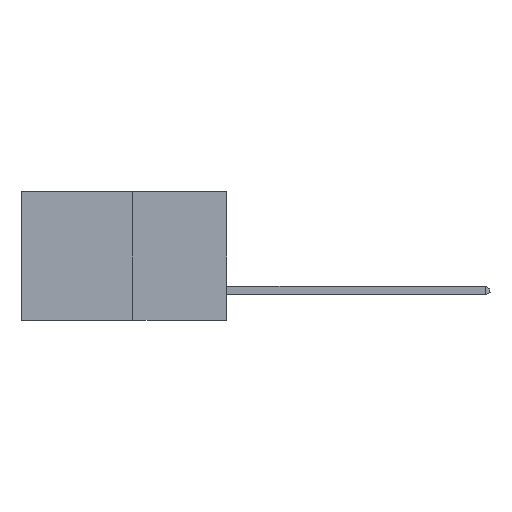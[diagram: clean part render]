
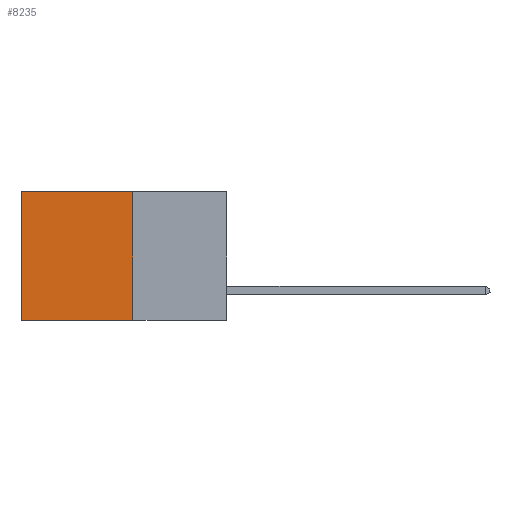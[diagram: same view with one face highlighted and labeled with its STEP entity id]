
A CAD part, left-side view. The second image highlights one B-rep face of the part: STEP entity #8235.
In plain terms, the highlighted planar face has unit normal (-1, 0, 0).
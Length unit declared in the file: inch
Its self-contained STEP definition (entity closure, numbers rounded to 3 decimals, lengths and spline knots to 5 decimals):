
#648 = LINE ( 'NONE', #4608, #25871 ) ;
#2080 = CARTESIAN_POINT ( 'NONE',  ( 0.277, 0.27, 0. ) ) ;
#4312 = VERTEX_POINT ( 'NONE', #30359 ) ;
#4608 = CARTESIAN_POINT ( 'NONE',  ( 0.277, 0.59, -0.37 ) ) ;
#6046 = PLANE ( 'NONE',  #11233 ) ;
#8235 = ADVANCED_FACE ( 'NONE', ( #15177 ), #6046, .F. ) ;
#8354 = EDGE_CURVE ( 'NONE', #21498, #4312, #23986, .T. ) ;
#8487 = DIRECTION ( 'NONE',  ( 1., 0., 0. ) ) ;
#8508 = CARTESIAN_POINT ( 'NONE',  ( 0.277, 0.27, -0.37 ) ) ;
#10447 = ORIENTED_EDGE ( 'NONE', *, *, #8354, .F. ) ;
#10821 = CARTESIAN_POINT ( 'NONE',  ( 0.277, 0.27, -0.37 ) ) ;
#10945 = DIRECTION ( 'NONE',  ( 0., 0., -1. ) ) ;
#11233 = AXIS2_PLACEMENT_3D ( 'NONE', #10821, #8487, #25065 ) ;
#15031 = LINE ( 'NONE', #8508, #26055 ) ;
#15131 = ORIENTED_EDGE ( 'NONE', *, *, #18727, .F. ) ;
#15177 = FACE_OUTER_BOUND ( 'NONE', #29595, .T. ) ;
#15483 = EDGE_CURVE ( 'NONE', #18466, #4312, #648, .T. ) ;
#17721 = VECTOR ( 'NONE', #23206, 39.37008 ) ;
#18173 = CARTESIAN_POINT ( 'NONE',  ( 0.277, 0.27, -0.37 ) ) ;
#18466 = VERTEX_POINT ( 'NONE', #21351 ) ;
#18663 = CARTESIAN_POINT ( 'NONE',  ( 0.277, 0.27, 0. ) ) ;
#18727 = EDGE_CURVE ( 'NONE', #25722, #21498, #15031, .T. ) ;
#20290 = ORIENTED_EDGE ( 'NONE', *, *, #20967, .T. ) ;
#20807 = CARTESIAN_POINT ( 'NONE',  ( 0.277, 0.27, -0.37 ) ) ;
#20967 = EDGE_CURVE ( 'NONE', #25722, #18466, #24357, .T. ) ;
#21221 = DIRECTION ( 'NONE',  ( 0., 0., -1. ) ) ;
#21351 = CARTESIAN_POINT ( 'NONE',  ( 0.277, 0.59, 0. ) ) ;
#21498 = VERTEX_POINT ( 'NONE', #18173 ) ;
#23206 = DIRECTION ( 'NONE',  ( 0., 1., 0. ) ) ;
#23986 = LINE ( 'NONE', #20807, #17721 ) ;
#24357 = LINE ( 'NONE', #18663, #30602 ) ;
#25065 = DIRECTION ( 'NONE',  ( 0., 0., -1. ) ) ;
#25722 = VERTEX_POINT ( 'NONE', #2080 ) ;
#25768 = DIRECTION ( 'NONE',  ( 0., 1., 0. ) ) ;
#25871 = VECTOR ( 'NONE', #21221, 39.37008 ) ;
#26055 = VECTOR ( 'NONE', #10945, 39.37008 ) ;
#29595 = EDGE_LOOP ( 'NONE', ( #30320, #10447, #15131, #20290 ) ) ;
#30320 = ORIENTED_EDGE ( 'NONE', *, *, #15483, .T. ) ;
#30359 = CARTESIAN_POINT ( 'NONE',  ( 0.277, 0.59, -0.37 ) ) ;
#30602 = VECTOR ( 'NONE', #25768, 39.37008 ) ;
